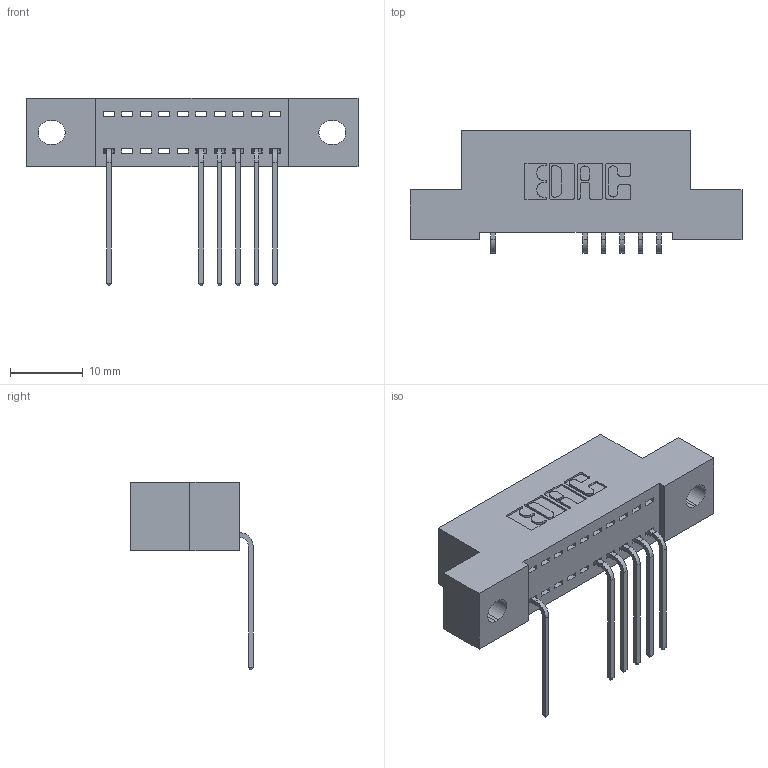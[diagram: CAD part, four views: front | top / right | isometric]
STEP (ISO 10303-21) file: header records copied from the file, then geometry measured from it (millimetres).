
FILE_DESCRIPTION (( 'STEP AP203' ), '1' );
FILE_NAME ('392-010-559-102.STEP', '2018-08-14T20:58:56', ( '' ), ( '' ), 'SwSTEP 2.0', 'SolidWorks 2016', '' );
FILE_SCHEMA (( 'CONFIG_CONTROL_DESIGN' ));
Length unit declared in the file: inch
Products named in the file (3): 342 Part_.128 Slot; 345-292-001_558 559 Tail - 1; 392-010-559-102
Assembly tree (7 placements, depth 2):
  392-010-559-102
    342 Part_.128 Slot
    345-292-001_558 559 Tail - 1  x6
Bounding box: 45.72 x 16.83 x 25.78 mm (x, y, z)
Volume: 3813 mm3; surface area: 4637.8 mm2
Topology: 7 solids, 7 shells, 522 faces, 1571 edges, 1038 vertices
Faces by surface type: plane 382, cylinder 140
Entity records: 10211 total; most frequent: CARTESIAN_POINT 1792, ORIENTED_EDGE 1742, DIRECTION 1571, EDGE_CURVE 871, LINE 743, VECTOR 743, VERTEX_POINT 578, AXIS2_PLACEMENT_3D 414
